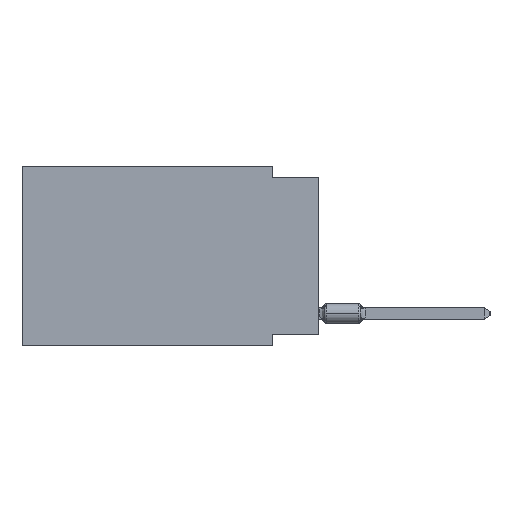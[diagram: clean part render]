
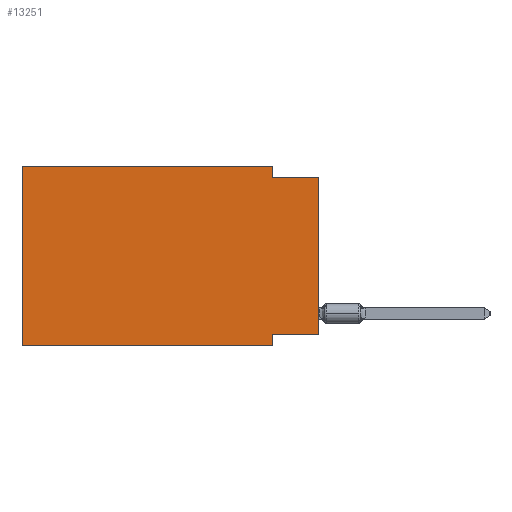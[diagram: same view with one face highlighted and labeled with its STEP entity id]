
A CAD part, left-side view. The second image highlights one B-rep face of the part: STEP entity #13251.
In plain terms, the highlighted planar face has unit normal (-1, 0, 0).
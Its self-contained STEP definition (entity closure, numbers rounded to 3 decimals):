
#613 = DIRECTION ( 'NONE',  ( 0., 1., 0. ) ) ;
#1651 = VECTOR ( 'NONE', #23962, 1000. ) ;
#3139 = ORIENTED_EDGE ( 'NONE', *, *, #28844, .F. ) ;
#4175 = CARTESIAN_POINT ( 'NONE',  ( 0., 2.54, -9.906 ) ) ;
#5392 = DIRECTION ( 'NONE',  ( 1., 0., 0. ) ) ;
#5479 = EDGE_CURVE ( 'NONE', #17520, #30816, #22176, .T. ) ;
#5979 = ORIENTED_EDGE ( 'NONE', *, *, #37395, .T. ) ;
#6264 = CARTESIAN_POINT ( 'NONE',  ( 0., 2.54, 0. ) ) ;
#6645 = VERTEX_POINT ( 'NONE', #33807 ) ;
#7865 = DIRECTION ( 'NONE',  ( 0., 0., -1. ) ) ;
#8959 = EDGE_CURVE ( 'NONE', #17520, #33767, #14592, .T. ) ;
#9857 = VERTEX_POINT ( 'NONE', #20688 ) ;
#10309 = CARTESIAN_POINT ( 'NONE',  ( 0., 16.383, 0. ) ) ;
#10874 = CARTESIAN_POINT ( 'NONE',  ( 0., 16.383, 0. ) ) ;
#11852 = EDGE_LOOP ( 'NONE', ( #5979, #16832, #36216, #27032, #41786, #34682, #39500, #3139 ) ) ;
#12529 = FACE_OUTER_BOUND ( 'NONE', #11852, .T. ) ;
#13251 = ADVANCED_FACE ( 'NONE', ( #12529 ), #19021, .F. ) ;
#14592 = LINE ( 'NONE', #26117, #32392 ) ;
#14755 = VERTEX_POINT ( 'NONE', #36882 ) ;
#16129 = LINE ( 'NONE', #36718, #35856 ) ;
#16832 = ORIENTED_EDGE ( 'NONE', *, *, #36942, .F. ) ;
#17520 = VERTEX_POINT ( 'NONE', #38873 ) ;
#17603 = CARTESIAN_POINT ( 'NONE',  ( 0., 0., -9.271 ) ) ;
#19021 = PLANE ( 'NONE',  #28642 ) ;
#20688 = CARTESIAN_POINT ( 'NONE',  ( 0., 2.54, -9.271 ) ) ;
#22176 = LINE ( 'NONE', #10874, #40294 ) ;
#23962 = DIRECTION ( 'NONE',  ( 0., -1., 0. ) ) ;
#24504 = EDGE_CURVE ( 'NONE', #43994, #14755, #25422, .T. ) ;
#24956 = CARTESIAN_POINT ( 'NONE',  ( 0., 2.54, 0. ) ) ;
#25422 = LINE ( 'NONE', #24956, #35554 ) ;
#25547 = EDGE_CURVE ( 'NONE', #30816, #43994, #34373, .T. ) ;
#26117 = CARTESIAN_POINT ( 'NONE',  ( 0., 16.383, -9.906 ) ) ;
#26761 = DIRECTION ( 'NONE',  ( 0., -1., 0. ) ) ;
#27032 = ORIENTED_EDGE ( 'NONE', *, *, #25547, .F. ) ;
#27860 = LINE ( 'NONE', #38964, #32813 ) ;
#28642 = AXIS2_PLACEMENT_3D ( 'NONE', #40041, #5392, #44179 ) ;
#28844 = EDGE_CURVE ( 'NONE', #39282, #9857, #27860, .T. ) ;
#29954 = LINE ( 'NONE', #40809, #34402 ) ;
#30816 = VERTEX_POINT ( 'NONE', #42501 ) ;
#31344 = VECTOR ( 'NONE', #31426, 1000. ) ;
#31426 = DIRECTION ( 'NONE',  ( 0., 0., -1. ) ) ;
#32145 = DIRECTION ( 'NONE',  ( 0., 0., 1. ) ) ;
#32392 = VECTOR ( 'NONE', #40214, 1000. ) ;
#32813 = VECTOR ( 'NONE', #613, 1000. ) ;
#33767 = VERTEX_POINT ( 'NONE', #34692 ) ;
#33807 = CARTESIAN_POINT ( 'NONE',  ( 0., 0., -0.635 ) ) ;
#34373 = LINE ( 'NONE', #10309, #1651 ) ;
#34402 = VECTOR ( 'NONE', #44043, 1000. ) ;
#34682 = ORIENTED_EDGE ( 'NONE', *, *, #8959, .T. ) ;
#34692 = CARTESIAN_POINT ( 'NONE',  ( 0., 2.54, -9.906 ) ) ;
#35554 = VECTOR ( 'NONE', #7865, 1000. ) ;
#35827 = LINE ( 'NONE', #4175, #31344 ) ;
#35856 = VECTOR ( 'NONE', #26761, 1000. ) ;
#36216 = ORIENTED_EDGE ( 'NONE', *, *, #24504, .F. ) ;
#36718 = CARTESIAN_POINT ( 'NONE',  ( 0., 0., -0.635 ) ) ;
#36882 = CARTESIAN_POINT ( 'NONE',  ( 0., 2.54, -0.635 ) ) ;
#36942 = EDGE_CURVE ( 'NONE', #14755, #6645, #16129, .T. ) ;
#37395 = EDGE_CURVE ( 'NONE', #39282, #6645, #29954, .T. ) ;
#38873 = CARTESIAN_POINT ( 'NONE',  ( 0., 16.383, -9.906 ) ) ;
#38964 = CARTESIAN_POINT ( 'NONE',  ( 0., 0., -9.271 ) ) ;
#39282 = VERTEX_POINT ( 'NONE', #17603 ) ;
#39500 = ORIENTED_EDGE ( 'NONE', *, *, #44128, .F. ) ;
#40041 = CARTESIAN_POINT ( 'NONE',  ( 0., 16.383, 0. ) ) ;
#40214 = DIRECTION ( 'NONE',  ( 0., -1., 0. ) ) ;
#40294 = VECTOR ( 'NONE', #32145, 1000. ) ;
#40809 = CARTESIAN_POINT ( 'NONE',  ( 0., 0., 0. ) ) ;
#41786 = ORIENTED_EDGE ( 'NONE', *, *, #5479, .F. ) ;
#42501 = CARTESIAN_POINT ( 'NONE',  ( 0., 16.383, 0. ) ) ;
#43994 = VERTEX_POINT ( 'NONE', #6264 ) ;
#44043 = DIRECTION ( 'NONE',  ( 0., 0., 1. ) ) ;
#44128 = EDGE_CURVE ( 'NONE', #9857, #33767, #35827, .T. ) ;
#44179 = DIRECTION ( 'NONE',  ( 0., 0., -1. ) ) ;
